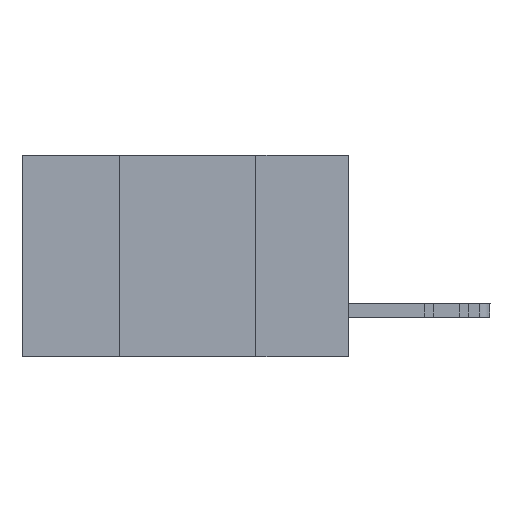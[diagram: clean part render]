
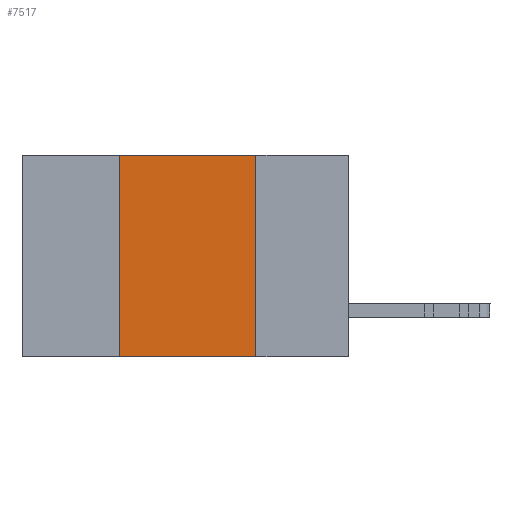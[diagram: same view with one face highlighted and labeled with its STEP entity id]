
A CAD part, left-side view. The second image highlights one B-rep face of the part: STEP entity #7517.
In plain terms, the highlighted planar face has unit normal (-1, 0, 0).
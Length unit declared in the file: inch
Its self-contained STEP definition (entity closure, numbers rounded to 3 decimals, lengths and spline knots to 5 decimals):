
#20 = VERTEX_POINT ( 'NONE', #24054 ) ;
#377 = EDGE_CURVE ( 'NONE', #23289, #11523, #4180, .T. ) ;
#404 = CARTESIAN_POINT ( 'NONE',  ( 0., 0.6, -0.37 ) ) ;
#1425 = VERTEX_POINT ( 'NONE', #14316 ) ;
#2228 = DIRECTION ( 'NONE',  ( 0., 0., 1. ) ) ;
#2485 = ORIENTED_EDGE ( 'NONE', *, *, #17896, .T. ) ;
#3234 = CARTESIAN_POINT ( 'NONE',  ( 0., 0.17, 0. ) ) ;
#4180 = LINE ( 'NONE', #24652, #19121 ) ;
#4752 = CARTESIAN_POINT ( 'NONE',  ( 0., 0.6, 0. ) ) ;
#6451 = ORIENTED_EDGE ( 'NONE', *, *, #19202, .F. ) ;
#6703 = DIRECTION ( 'NONE',  ( 1., 0., 0. ) ) ;
#7517 = ADVANCED_FACE ( 'NONE', ( #11578 ), #16421, .F. ) ;
#9202 = CARTESIAN_POINT ( 'NONE',  ( 0., 0.17, -0.37 ) ) ;
#10186 = DIRECTION ( 'NONE',  ( 0., -1., 0. ) ) ;
#11153 = DIRECTION ( 'NONE',  ( 0., 0., -1. ) ) ;
#11342 = EDGE_LOOP ( 'NONE', ( #12921, #12874, #6451, #2485 ) ) ;
#11523 = VERTEX_POINT ( 'NONE', #9202 ) ;
#11578 = FACE_OUTER_BOUND ( 'NONE', #11342, .T. ) ;
#12046 = CARTESIAN_POINT ( 'NONE',  ( 0., 0.42, -0.37 ) ) ;
#12825 = VECTOR ( 'NONE', #2228, 39.37008 ) ;
#12874 = ORIENTED_EDGE ( 'NONE', *, *, #20505, .F. ) ;
#12921 = ORIENTED_EDGE ( 'NONE', *, *, #377, .F. ) ;
#13929 = VECTOR ( 'NONE', #10186, 39.37008 ) ;
#14316 = CARTESIAN_POINT ( 'NONE',  ( 0., 0.42, 0. ) ) ;
#16421 = PLANE ( 'NONE',  #20374 ) ;
#17896 = EDGE_CURVE ( 'NONE', #20, #11523, #23757, .T. ) ;
#18627 = VECTOR ( 'NONE', #23760, 39.37008 ) ;
#19121 = VECTOR ( 'NONE', #11153, 39.37008 ) ;
#19202 = EDGE_CURVE ( 'NONE', #20, #1425, #23093, .T. ) ;
#19845 = CARTESIAN_POINT ( 'NONE',  ( 0., 0.6, 0. ) ) ;
#20317 = DIRECTION ( 'NONE',  ( 0., 0., -1. ) ) ;
#20374 = AXIS2_PLACEMENT_3D ( 'NONE', #4752, #6703, #20317 ) ;
#20505 = EDGE_CURVE ( 'NONE', #1425, #23289, #24188, .T. ) ;
#23093 = LINE ( 'NONE', #12046, #12825 ) ;
#23289 = VERTEX_POINT ( 'NONE', #3234 ) ;
#23757 = LINE ( 'NONE', #404, #18627 ) ;
#23760 = DIRECTION ( 'NONE',  ( 0., -1., 0. ) ) ;
#24054 = CARTESIAN_POINT ( 'NONE',  ( 0., 0.42, -0.37 ) ) ;
#24188 = LINE ( 'NONE', #19845, #13929 ) ;
#24652 = CARTESIAN_POINT ( 'NONE',  ( 0., 0.17, -0.37 ) ) ;
